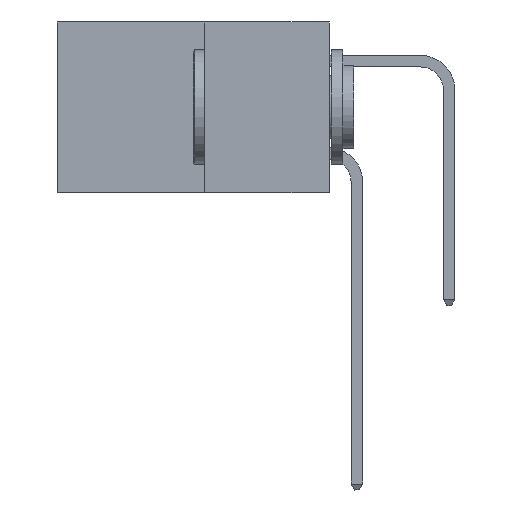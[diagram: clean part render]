
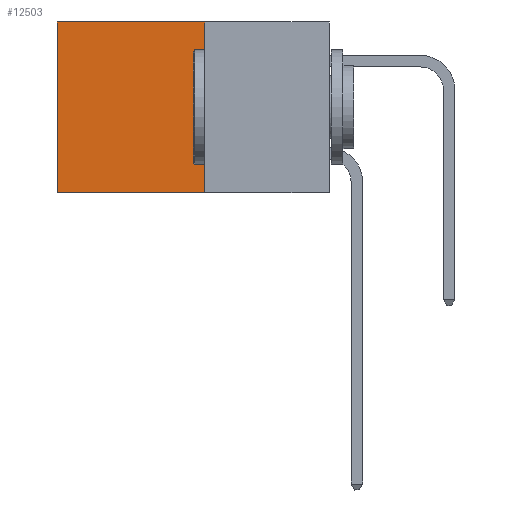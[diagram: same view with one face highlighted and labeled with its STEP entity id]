
A CAD part, left-side view. The second image highlights one B-rep face of the part: STEP entity #12503.
In plain terms, the highlighted planar face has unit normal (-1, 0, 0).
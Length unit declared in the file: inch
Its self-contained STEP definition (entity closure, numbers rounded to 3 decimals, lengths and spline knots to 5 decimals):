
#1710 = CARTESIAN_POINT ( 'NONE',  ( 0.277, 0.27, -0.37 ) ) ;
#1787 = EDGE_CURVE ( 'NONE', #18493, #20394, #14285, .T. ) ;
#1886 = DIRECTION ( 'NONE',  ( 0., 1., 0. ) ) ;
#2150 = VECTOR ( 'NONE', #12315, 39.37008 ) ;
#3384 = DIRECTION ( 'NONE',  ( 0., 0., -1. ) ) ;
#4071 = EDGE_CURVE ( 'NONE', #6485, #20394, #9766, .T. ) ;
#5349 = EDGE_CURVE ( 'NONE', #11665, #18493, #17719, .T. ) ;
#5433 = VECTOR ( 'NONE', #8212, 39.37008 ) ;
#6485 = VERTEX_POINT ( 'NONE', #16648 ) ;
#7099 = ORIENTED_EDGE ( 'NONE', *, *, #9499, .F. ) ;
#7673 = LINE ( 'NONE', #9631, #2150 ) ;
#8212 = DIRECTION ( 'NONE',  ( 0., 0., -1. ) ) ;
#8273 = EDGE_LOOP ( 'NONE', ( #20123, #17076, #7099, #8899 ) ) ;
#8899 = ORIENTED_EDGE ( 'NONE', *, *, #5349, .T. ) ;
#9499 = EDGE_CURVE ( 'NONE', #11665, #6485, #7673, .T. ) ;
#9631 = CARTESIAN_POINT ( 'NONE',  ( 0.277, 0.27, -0.37 ) ) ;
#9766 = LINE ( 'NONE', #18741, #18080 ) ;
#10061 = PLANE ( 'NONE',  #13129 ) ;
#10521 = CARTESIAN_POINT ( 'NONE',  ( 0.277, 0.59, -0.37 ) ) ;
#11665 = VERTEX_POINT ( 'NONE', #14666 ) ;
#12315 = DIRECTION ( 'NONE',  ( 0., 0., -1. ) ) ;
#12503 = ADVANCED_FACE ( 'NONE', ( #20090 ), #10061, .F. ) ;
#13129 = AXIS2_PLACEMENT_3D ( 'NONE', #1710, #13410, #3384 ) ;
#13410 = DIRECTION ( 'NONE',  ( 1., 0., 0. ) ) ;
#14285 = LINE ( 'NONE', #10521, #5433 ) ;
#14435 = CARTESIAN_POINT ( 'NONE',  ( 0.277, 0.59, 0. ) ) ;
#14666 = CARTESIAN_POINT ( 'NONE',  ( 0.277, 0.27, 0. ) ) ;
#16648 = CARTESIAN_POINT ( 'NONE',  ( 0.277, 0.27, -0.37 ) ) ;
#17076 = ORIENTED_EDGE ( 'NONE', *, *, #4071, .F. ) ;
#17719 = LINE ( 'NONE', #18473, #20610 ) ;
#17990 = CARTESIAN_POINT ( 'NONE',  ( 0.277, 0.59, -0.37 ) ) ;
#18080 = VECTOR ( 'NONE', #18787, 39.37008 ) ;
#18473 = CARTESIAN_POINT ( 'NONE',  ( 0.277, 0.27, 0. ) ) ;
#18493 = VERTEX_POINT ( 'NONE', #14435 ) ;
#18741 = CARTESIAN_POINT ( 'NONE',  ( 0.277, 0.27, -0.37 ) ) ;
#18787 = DIRECTION ( 'NONE',  ( 0., 1., 0. ) ) ;
#20090 = FACE_OUTER_BOUND ( 'NONE', #8273, .T. ) ;
#20123 = ORIENTED_EDGE ( 'NONE', *, *, #1787, .T. ) ;
#20394 = VERTEX_POINT ( 'NONE', #17990 ) ;
#20610 = VECTOR ( 'NONE', #1886, 39.37008 ) ;
